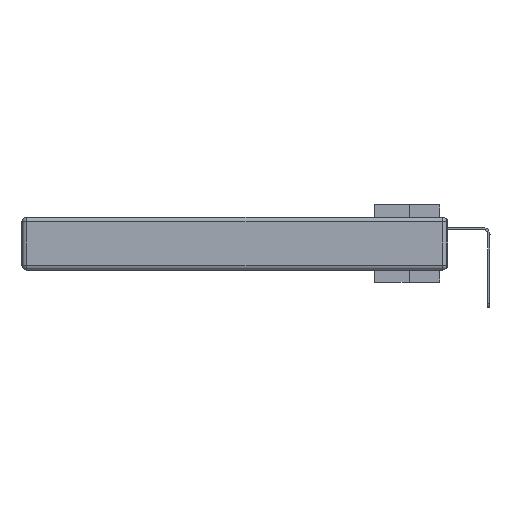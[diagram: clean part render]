
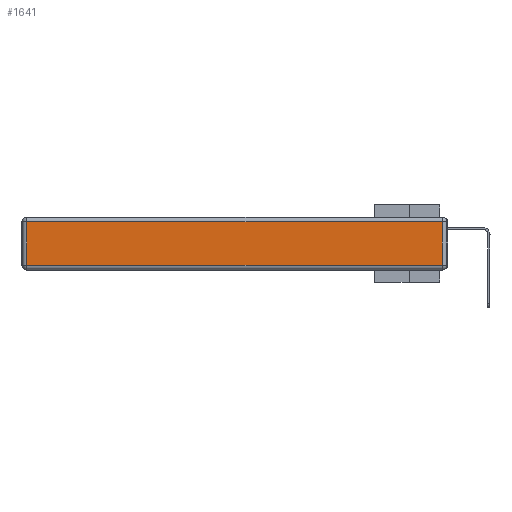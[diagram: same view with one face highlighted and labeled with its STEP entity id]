
A CAD part, left-side view. The second image highlights one B-rep face of the part: STEP entity #1641.
In plain terms, the highlighted planar face has unit normal (-1, 0, 0).
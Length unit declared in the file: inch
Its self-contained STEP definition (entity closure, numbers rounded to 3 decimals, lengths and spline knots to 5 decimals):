
#1641 = ADVANCED_FACE ( 'NONE', ( #3364 ), #18416, .T. ) ;
#1895 = DIRECTION ( 'NONE',  ( -1., 0., 0. ) ) ;
#2372 = EDGE_CURVE ( 'NONE', #35515, #26102, #7609, .T. ) ;
#3364 = FACE_OUTER_BOUND ( 'NONE', #25529, .T. ) ;
#4435 = DIRECTION ( 'NONE',  ( 0., 0., 1. ) ) ;
#6809 = LINE ( 'NONE', #26575, #33306 ) ;
#7429 = DIRECTION ( 'NONE',  ( 0., 0., 1. ) ) ;
#7609 = LINE ( 'NONE', #24670, #14072 ) ;
#7964 = ORIENTED_EDGE ( 'NONE', *, *, #23825, .T. ) ;
#12680 = ORIENTED_EDGE ( 'NONE', *, *, #2372, .T. ) ;
#13262 = ORIENTED_EDGE ( 'NONE', *, *, #20767, .T. ) ;
#13349 = DIRECTION ( 'NONE',  ( 0., 0., -1. ) ) ;
#13583 = CARTESIAN_POINT ( 'NONE',  ( 0., 0., -0.343 ) ) ;
#14072 = VECTOR ( 'NONE', #30510, 39.37008 ) ;
#16710 = VECTOR ( 'NONE', #30698, 39.37008 ) ;
#18046 = CARTESIAN_POINT ( 'NONE',  ( 0., 2.72, -0.313 ) ) ;
#18416 = PLANE ( 'NONE',  #26405 ) ;
#18702 = VERTEX_POINT ( 'NONE', #33264 ) ;
#20767 = EDGE_CURVE ( 'NONE', #18702, #29114, #25838, .T. ) ;
#21680 = VECTOR ( 'NONE', #13349, 39.37008 ) ;
#22237 = CARTESIAN_POINT ( 'NONE',  ( 0., 2.72, -0.03 ) ) ;
#23825 = EDGE_CURVE ( 'NONE', #26102, #18702, #6809, .T. ) ;
#24154 = CARTESIAN_POINT ( 'NONE',  ( 0., 2.72, -0.343 ) ) ;
#24670 = CARTESIAN_POINT ( 'NONE',  ( 0., 0., -0.313 ) ) ;
#25529 = EDGE_LOOP ( 'NONE', ( #12680, #7964, #13262, #31814 ) ) ;
#25838 = LINE ( 'NONE', #27899, #16710 ) ;
#26102 = VERTEX_POINT ( 'NONE', #29212 ) ;
#26405 = AXIS2_PLACEMENT_3D ( 'NONE', #13583, #1895, #4435 ) ;
#26575 = CARTESIAN_POINT ( 'NONE',  ( 0., 0.03, -0.343 ) ) ;
#27667 = EDGE_CURVE ( 'NONE', #29114, #35515, #32972, .T. ) ;
#27899 = CARTESIAN_POINT ( 'NONE',  ( 0., 2.75, -0.03 ) ) ;
#29114 = VERTEX_POINT ( 'NONE', #22237 ) ;
#29212 = CARTESIAN_POINT ( 'NONE',  ( 0., 0.03, -0.313 ) ) ;
#30510 = DIRECTION ( 'NONE',  ( 0., -1., 0. ) ) ;
#30698 = DIRECTION ( 'NONE',  ( 0., 1., 0. ) ) ;
#31814 = ORIENTED_EDGE ( 'NONE', *, *, #27667, .T. ) ;
#32972 = LINE ( 'NONE', #24154, #21680 ) ;
#33264 = CARTESIAN_POINT ( 'NONE',  ( 0., 0.03, -0.03 ) ) ;
#33306 = VECTOR ( 'NONE', #7429, 39.37008 ) ;
#35515 = VERTEX_POINT ( 'NONE', #18046 ) ;
